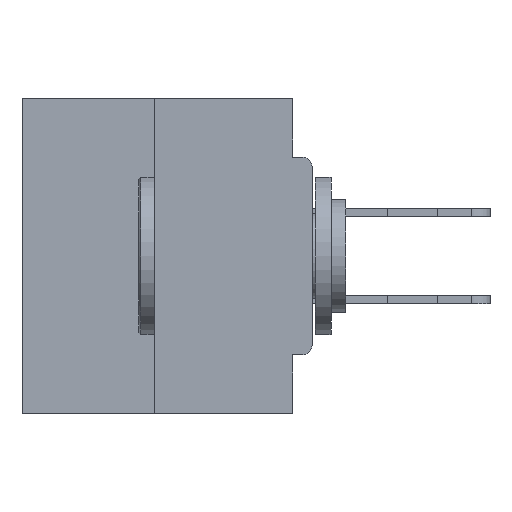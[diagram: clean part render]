
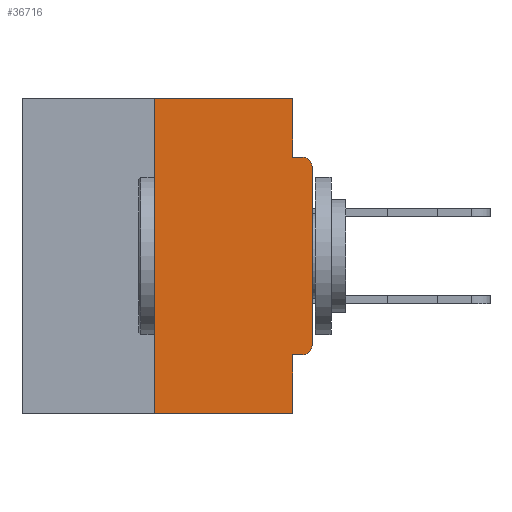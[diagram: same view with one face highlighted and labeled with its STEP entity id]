
A CAD part, left-side view. The second image highlights one B-rep face of the part: STEP entity #36716.
In plain terms, the highlighted planar face has unit normal (-1, 0, 0).
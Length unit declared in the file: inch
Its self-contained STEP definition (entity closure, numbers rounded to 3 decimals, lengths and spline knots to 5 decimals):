
#259 = ORIENTED_EDGE ( 'NONE', *, *, #26724, .F. ) ;
#780 = VERTEX_POINT ( 'NONE', #35356 ) ;
#1232 = CARTESIAN_POINT ( 'NONE',  ( 0., 0.031, -0.5 ) ) ;
#1425 = VECTOR ( 'NONE', #17405, 39.37008 ) ;
#1889 = EDGE_CURVE ( 'NONE', #5346, #19029, #33884, .T. ) ;
#3051 = CIRCLE ( 'NONE', #19986, 0.015 ) ;
#4120 = LINE ( 'NONE', #8387, #16145 ) ;
#4619 = DIRECTION ( 'NONE',  ( 0., 0., -1. ) ) ;
#4945 = CARTESIAN_POINT ( 'NONE',  ( 0., 0.46, 0. ) ) ;
#5244 = ORIENTED_EDGE ( 'NONE', *, *, #25254, .F. ) ;
#5336 = ORIENTED_EDGE ( 'NONE', *, *, #24062, .F. ) ;
#5346 = VERTEX_POINT ( 'NONE', #21168 ) ;
#6675 = CIRCLE ( 'NONE', #13615, 0.015 ) ;
#7117 = VECTOR ( 'NONE', #28538, 39.37008 ) ;
#7276 = DIRECTION ( 'NONE',  ( 1., 0., 0. ) ) ;
#7395 = FACE_OUTER_BOUND ( 'NONE', #14608, .T. ) ;
#7513 = DIRECTION ( 'NONE',  ( 0., 0., -1. ) ) ;
#8022 = CARTESIAN_POINT ( 'NONE',  ( 0., 0.25, 0. ) ) ;
#8387 = CARTESIAN_POINT ( 'NONE',  ( 0., 0., 0. ) ) ;
#8505 = CARTESIAN_POINT ( 'NONE',  ( 0., 0., -0.0935 ) ) ;
#9097 = LINE ( 'NONE', #12525, #23821 ) ;
#10143 = VERTEX_POINT ( 'NONE', #30123 ) ;
#10266 = CARTESIAN_POINT ( 'NONE',  ( 0., 0.015, -0.4065 ) ) ;
#10277 = DIRECTION ( 'NONE',  ( 0., 0., -1. ) ) ;
#10765 = VERTEX_POINT ( 'NONE', #18117 ) ;
#11031 = EDGE_CURVE ( 'NONE', #33811, #5346, #17952, .T. ) ;
#11152 = DIRECTION ( 'NONE',  ( 0., -1., 0. ) ) ;
#12083 = EDGE_CURVE ( 'NONE', #10765, #22162, #12903, .T. ) ;
#12525 = CARTESIAN_POINT ( 'NONE',  ( 0., 0.46, 0. ) ) ;
#12903 = LINE ( 'NONE', #31142, #7117 ) ;
#13462 = EDGE_CURVE ( 'NONE', #29675, #28439, #3051, .T. ) ;
#13615 = AXIS2_PLACEMENT_3D ( 'NONE', #32963, #24143, #10277 ) ;
#14608 = EDGE_LOOP ( 'NONE', ( #5336, #36961, #15912, #33608, #29586, #35805, #34032, #16691, #259, #5244 ) ) ;
#15898 = PLANE ( 'NONE',  #32776 ) ;
#15912 = ORIENTED_EDGE ( 'NONE', *, *, #22358, .T. ) ;
#16145 = VECTOR ( 'NONE', #31100, 39.37008 ) ;
#16397 = VERTEX_POINT ( 'NONE', #31121 ) ;
#16672 = LINE ( 'NONE', #28663, #17591 ) ;
#16691 = ORIENTED_EDGE ( 'NONE', *, *, #13462, .T. ) ;
#16896 = CARTESIAN_POINT ( 'NONE',  ( 0., 0.031, 0. ) ) ;
#17316 = DIRECTION ( 'NONE',  ( 0., -1., 0. ) ) ;
#17405 = DIRECTION ( 'NONE',  ( 0., 0., -1. ) ) ;
#17491 = LINE ( 'NONE', #16896, #1425 ) ;
#17591 = VECTOR ( 'NONE', #17316, 39.37008 ) ;
#17952 = LINE ( 'NONE', #20395, #22826 ) ;
#18117 = CARTESIAN_POINT ( 'NONE',  ( 0., 0.25, -0.5 ) ) ;
#19029 = VERTEX_POINT ( 'NONE', #1232 ) ;
#19400 = CARTESIAN_POINT ( 'NONE',  ( 0., 0.015, -0.0935 ) ) ;
#19566 = LINE ( 'NONE', #8505, #25344 ) ;
#19986 = AXIS2_PLACEMENT_3D ( 'NONE', #22146, #25033, #4619 ) ;
#20395 = CARTESIAN_POINT ( 'NONE',  ( 0., 0., -0.4065 ) ) ;
#21168 = CARTESIAN_POINT ( 'NONE',  ( 0., 0.031, -0.4065 ) ) ;
#22146 = CARTESIAN_POINT ( 'NONE',  ( 0., 0.015, -0.1085 ) ) ;
#22162 = VERTEX_POINT ( 'NONE', #8022 ) ;
#22358 = EDGE_CURVE ( 'NONE', #10765, #19029, #16672, .T. ) ;
#22826 = VECTOR ( 'NONE', #23263, 39.37008 ) ;
#23263 = DIRECTION ( 'NONE',  ( 0., 1., 0. ) ) ;
#23821 = VECTOR ( 'NONE', #32349, 39.37008 ) ;
#24062 = EDGE_CURVE ( 'NONE', #22162, #16397, #9097, .T. ) ;
#24143 = DIRECTION ( 'NONE',  ( -1., 0., 0. ) ) ;
#25033 = DIRECTION ( 'NONE',  ( -1., 0., 0. ) ) ;
#25254 = EDGE_CURVE ( 'NONE', #16397, #10143, #17491, .T. ) ;
#25298 = EDGE_CURVE ( 'NONE', #780, #29675, #4120, .T. ) ;
#25344 = VECTOR ( 'NONE', #11152, 39.37008 ) ;
#26310 = VECTOR ( 'NONE', #33140, 39.37008 ) ;
#26724 = EDGE_CURVE ( 'NONE', #10143, #28439, #19566, .T. ) ;
#28315 = CARTESIAN_POINT ( 'NONE',  ( 0., 0., -0.1085 ) ) ;
#28439 = VERTEX_POINT ( 'NONE', #19400 ) ;
#28538 = DIRECTION ( 'NONE',  ( 0., 0., 1. ) ) ;
#28663 = CARTESIAN_POINT ( 'NONE',  ( 0., 0.46, -0.5 ) ) ;
#29586 = ORIENTED_EDGE ( 'NONE', *, *, #11031, .F. ) ;
#29675 = VERTEX_POINT ( 'NONE', #28315 ) ;
#30123 = CARTESIAN_POINT ( 'NONE',  ( 0., 0.031, -0.0935 ) ) ;
#31100 = DIRECTION ( 'NONE',  ( 0., 0., 1. ) ) ;
#31121 = CARTESIAN_POINT ( 'NONE',  ( 0., 0.031, 0. ) ) ;
#31142 = CARTESIAN_POINT ( 'NONE',  ( 0., 0.25, 0. ) ) ;
#32349 = DIRECTION ( 'NONE',  ( 0., -1., 0. ) ) ;
#32776 = AXIS2_PLACEMENT_3D ( 'NONE', #4945, #7276, #7513 ) ;
#32963 = CARTESIAN_POINT ( 'NONE',  ( 0., 0.015, -0.3915 ) ) ;
#33140 = DIRECTION ( 'NONE',  ( 0., 0., -1. ) ) ;
#33608 = ORIENTED_EDGE ( 'NONE', *, *, #1889, .F. ) ;
#33811 = VERTEX_POINT ( 'NONE', #10266 ) ;
#33884 = LINE ( 'NONE', #36412, #26310 ) ;
#34032 = ORIENTED_EDGE ( 'NONE', *, *, #25298, .T. ) ;
#34831 = EDGE_CURVE ( 'NONE', #33811, #780, #6675, .T. ) ;
#35356 = CARTESIAN_POINT ( 'NONE',  ( 0., 0., -0.3915 ) ) ;
#35805 = ORIENTED_EDGE ( 'NONE', *, *, #34831, .T. ) ;
#36412 = CARTESIAN_POINT ( 'NONE',  ( 0., 0.031, -0.5 ) ) ;
#36716 = ADVANCED_FACE ( 'NONE', ( #7395 ), #15898, .F. ) ;
#36961 = ORIENTED_EDGE ( 'NONE', *, *, #12083, .F. ) ;
